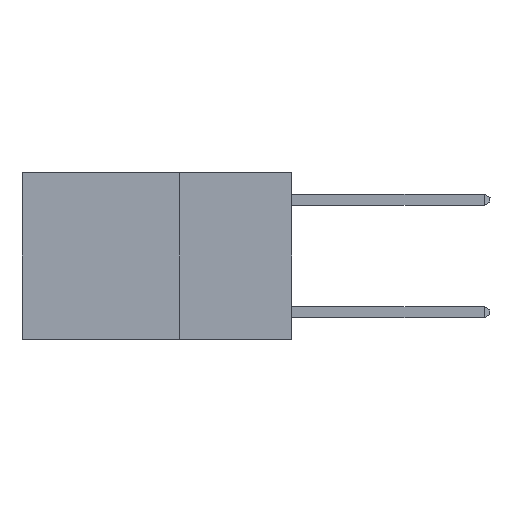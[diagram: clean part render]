
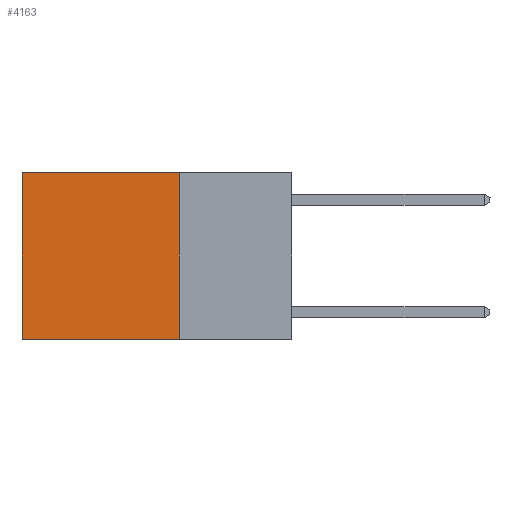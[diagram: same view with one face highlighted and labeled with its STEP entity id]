
A CAD part, left-side view. The second image highlights one B-rep face of the part: STEP entity #4163.
In plain terms, the highlighted planar face has unit normal (-1, 0, 0).
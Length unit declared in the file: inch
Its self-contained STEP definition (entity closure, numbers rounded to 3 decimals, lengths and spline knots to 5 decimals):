
#346 = DIRECTION ( 'NONE',  ( 0., 0., -1. ) ) ;
#381 = VERTEX_POINT ( 'NONE', #6173 ) ;
#3628 = VECTOR ( 'NONE', #4736, 39.37008 ) ;
#4163 = ADVANCED_FACE ( 'NONE', ( #13347 ), #21433, .F. ) ;
#4677 = VECTOR ( 'NONE', #346, 39.37008 ) ;
#4736 = DIRECTION ( 'NONE',  ( 0., 0., -1. ) ) ;
#4928 = DIRECTION ( 'NONE',  ( 0., 1., 0. ) ) ;
#5750 = EDGE_CURVE ( 'NONE', #18985, #381, #10133, .T. ) ;
#6173 = CARTESIAN_POINT ( 'NONE',  ( 0.2625, 0.6, -0.37 ) ) ;
#8210 = VERTEX_POINT ( 'NONE', #14272 ) ;
#8249 = EDGE_LOOP ( 'NONE', ( #23534, #17982, #20928, #21900 ) ) ;
#9323 = LINE ( 'NONE', #12348, #4677 ) ;
#9430 = CARTESIAN_POINT ( 'NONE',  ( 0.2625, 0.25, -0.37 ) ) ;
#10133 = LINE ( 'NONE', #18531, #3628 ) ;
#10585 = LINE ( 'NONE', #24459, #15255 ) ;
#10914 = VECTOR ( 'NONE', #23999, 39.37008 ) ;
#11539 = LINE ( 'NONE', #14321, #10914 ) ;
#11745 = DIRECTION ( 'NONE',  ( 1., 0., 0. ) ) ;
#11847 = EDGE_CURVE ( 'NONE', #8210, #18985, #11539, .T. ) ;
#12348 = CARTESIAN_POINT ( 'NONE',  ( 0.2625, 0.25, 0. ) ) ;
#13347 = FACE_OUTER_BOUND ( 'NONE', #8249, .T. ) ;
#14272 = CARTESIAN_POINT ( 'NONE',  ( 0.2625, 0.25, 0. ) ) ;
#14321 = CARTESIAN_POINT ( 'NONE',  ( 0.2625, 0.25, 0. ) ) ;
#15255 = VECTOR ( 'NONE', #4928, 39.37008 ) ;
#15406 = CARTESIAN_POINT ( 'NONE',  ( 0.2625, 0.6, 0. ) ) ;
#16306 = VERTEX_POINT ( 'NONE', #9430 ) ;
#16677 = EDGE_CURVE ( 'NONE', #16306, #381, #10585, .T. ) ;
#17902 = EDGE_CURVE ( 'NONE', #8210, #16306, #9323, .T. ) ;
#17982 = ORIENTED_EDGE ( 'NONE', *, *, #16677, .F. ) ;
#18391 = AXIS2_PLACEMENT_3D ( 'NONE', #23446, #11745, #25346 ) ;
#18531 = CARTESIAN_POINT ( 'NONE',  ( 0.2625, 0.6, 0. ) ) ;
#18985 = VERTEX_POINT ( 'NONE', #15406 ) ;
#20928 = ORIENTED_EDGE ( 'NONE', *, *, #17902, .F. ) ;
#21433 = PLANE ( 'NONE',  #18391 ) ;
#21900 = ORIENTED_EDGE ( 'NONE', *, *, #11847, .T. ) ;
#23446 = CARTESIAN_POINT ( 'NONE',  ( 0.2625, 0.25, 0. ) ) ;
#23534 = ORIENTED_EDGE ( 'NONE', *, *, #5750, .T. ) ;
#23999 = DIRECTION ( 'NONE',  ( 0., 1., 0. ) ) ;
#24459 = CARTESIAN_POINT ( 'NONE',  ( 0.2625, 0.25, -0.37 ) ) ;
#25346 = DIRECTION ( 'NONE',  ( 0., 0., -1. ) ) ;
